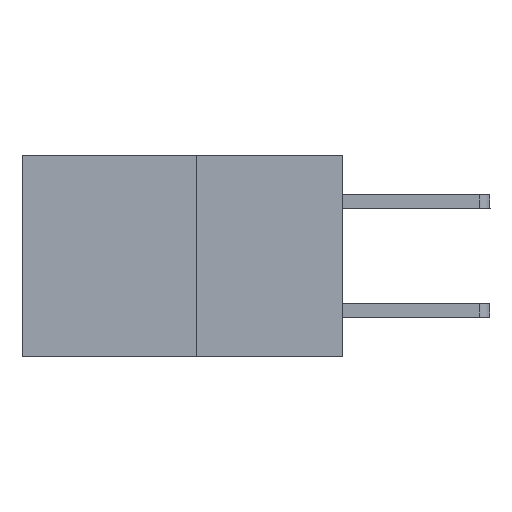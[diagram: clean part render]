
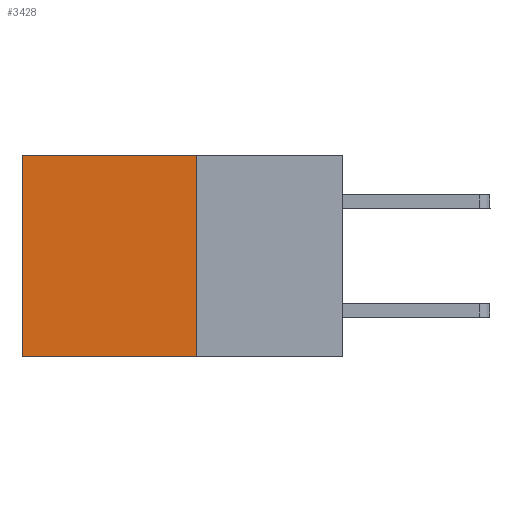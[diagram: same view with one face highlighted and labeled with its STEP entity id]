
A CAD part, left-side view. The second image highlights one B-rep face of the part: STEP entity #3428.
In plain terms, the highlighted planar face has unit normal (-1, 0, 0).
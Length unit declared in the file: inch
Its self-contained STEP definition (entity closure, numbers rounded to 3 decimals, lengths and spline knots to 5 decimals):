
#445 = CARTESIAN_POINT ( 'NONE',  ( 0.277, 0.59, 0. ) ) ;
#1346 = CARTESIAN_POINT ( 'NONE',  ( 0.277, 0.59, -0.37 ) ) ;
#1496 = CARTESIAN_POINT ( 'NONE',  ( 0.277, 0.27, -0.37 ) ) ;
#1748 = FACE_OUTER_BOUND ( 'NONE', #3253, .T. ) ;
#2135 = VECTOR ( 'NONE', #5916, 39.37008 ) ;
#2341 = LINE ( 'NONE', #5516, #2135 ) ;
#2395 = VECTOR ( 'NONE', #5384, 39.37008 ) ;
#2552 = EDGE_CURVE ( 'NONE', #2709, #5344, #8543, .T. ) ;
#2709 = VERTEX_POINT ( 'NONE', #7279 ) ;
#2916 = CARTESIAN_POINT ( 'NONE',  ( 0.277, 0.27, -0.37 ) ) ;
#2921 = DIRECTION ( 'NONE',  ( 0., 0., -1. ) ) ;
#2993 = ORIENTED_EDGE ( 'NONE', *, *, #3363, .F. ) ;
#3203 = ORIENTED_EDGE ( 'NONE', *, *, #5547, .F. ) ;
#3253 = EDGE_LOOP ( 'NONE', ( #7641, #3203, #2993, #3866 ) ) ;
#3363 = EDGE_CURVE ( 'NONE', #2709, #4554, #7811, .T. ) ;
#3428 = ADVANCED_FACE ( 'NONE', ( #1748 ), #4750, .F. ) ;
#3581 = VERTEX_POINT ( 'NONE', #5636 ) ;
#3866 = ORIENTED_EDGE ( 'NONE', *, *, #2552, .T. ) ;
#3924 = LINE ( 'NONE', #1346, #5405 ) ;
#4554 = VERTEX_POINT ( 'NONE', #1496 ) ;
#4750 = PLANE ( 'NONE',  #7575 ) ;
#5121 = DIRECTION ( 'NONE',  ( 0., 0., -1. ) ) ;
#5344 = VERTEX_POINT ( 'NONE', #445 ) ;
#5384 = DIRECTION ( 'NONE',  ( 0., 0., -1. ) ) ;
#5405 = VECTOR ( 'NONE', #2921, 39.37008 ) ;
#5516 = CARTESIAN_POINT ( 'NONE',  ( 0.277, 0.27, -0.37 ) ) ;
#5547 = EDGE_CURVE ( 'NONE', #4554, #3581, #2341, .T. ) ;
#5588 = DIRECTION ( 'NONE',  ( 0., 1., 0. ) ) ;
#5636 = CARTESIAN_POINT ( 'NONE',  ( 0.277, 0.59, -0.37 ) ) ;
#5916 = DIRECTION ( 'NONE',  ( 0., 1., 0. ) ) ;
#6545 = CARTESIAN_POINT ( 'NONE',  ( 0.277, 0.27, -0.37 ) ) ;
#6745 = VECTOR ( 'NONE', #5588, 39.37008 ) ;
#7114 = CARTESIAN_POINT ( 'NONE',  ( 0.277, 0.27, 0. ) ) ;
#7279 = CARTESIAN_POINT ( 'NONE',  ( 0.277, 0.27, 0. ) ) ;
#7575 = AXIS2_PLACEMENT_3D ( 'NONE', #6545, #8716, #5121 ) ;
#7641 = ORIENTED_EDGE ( 'NONE', *, *, #7742, .T. ) ;
#7742 = EDGE_CURVE ( 'NONE', #5344, #3581, #3924, .T. ) ;
#7811 = LINE ( 'NONE', #2916, #2395 ) ;
#8543 = LINE ( 'NONE', #7114, #6745 ) ;
#8716 = DIRECTION ( 'NONE',  ( 1., 0., 0. ) ) ;
